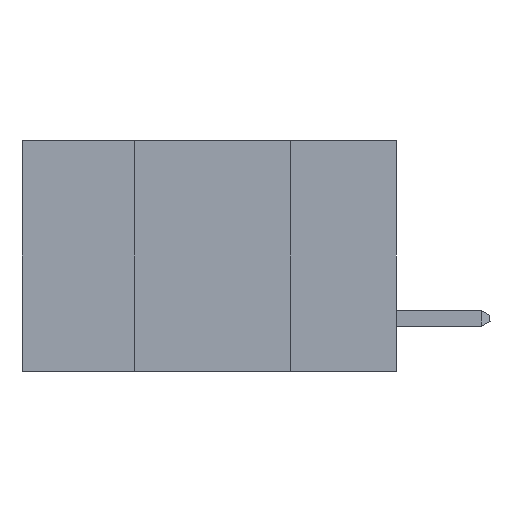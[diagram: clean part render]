
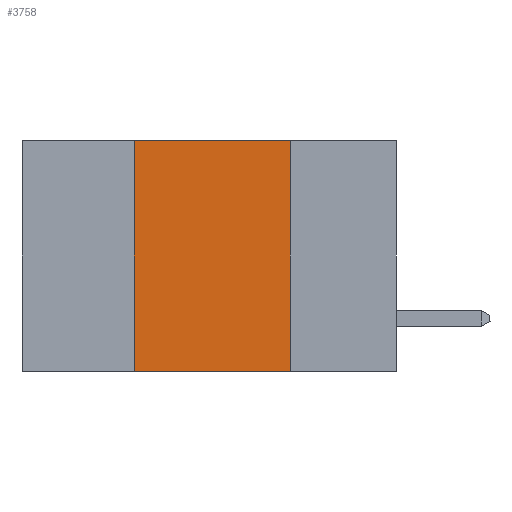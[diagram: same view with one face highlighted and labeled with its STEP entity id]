
A CAD part, left-side view. The second image highlights one B-rep face of the part: STEP entity #3758.
In plain terms, the highlighted planar face has unit normal (-1, 0, 0).
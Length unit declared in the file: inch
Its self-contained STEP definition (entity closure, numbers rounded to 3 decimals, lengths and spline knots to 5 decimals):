
#386 = LINE ( 'NONE', #14880, #13480 ) ;
#495 = DIRECTION ( 'NONE',  ( 0., 0., 1. ) ) ;
#1566 = VECTOR ( 'NONE', #15967, 39.37008 ) ;
#2163 = DIRECTION ( 'NONE',  ( 0., -1., 0. ) ) ;
#2364 = VECTOR ( 'NONE', #2163, 39.37008 ) ;
#2517 = EDGE_LOOP ( 'NONE', ( #6542, #15307, #7338, #2633 ) ) ;
#2633 = ORIENTED_EDGE ( 'NONE', *, *, #7974, .T. ) ;
#3292 = DIRECTION ( 'NONE',  ( 1., 0., 0. ) ) ;
#3332 = VERTEX_POINT ( 'NONE', #13618 ) ;
#3379 = DIRECTION ( 'NONE',  ( 0., 0., -1. ) ) ;
#3758 = ADVANCED_FACE ( 'NONE', ( #7719 ), #9245, .F. ) ;
#4169 = VERTEX_POINT ( 'NONE', #14864 ) ;
#4485 = CARTESIAN_POINT ( 'NONE',  ( 0., 0.6, 0. ) ) ;
#4573 = CARTESIAN_POINT ( 'NONE',  ( 0., 0.17, 0. ) ) ;
#5188 = EDGE_CURVE ( 'NONE', #4169, #11211, #386, .T. ) ;
#5223 = CARTESIAN_POINT ( 'NONE',  ( 0., 0.42, 0. ) ) ;
#6510 = CARTESIAN_POINT ( 'NONE',  ( 0., 0.6, 0. ) ) ;
#6542 = ORIENTED_EDGE ( 'NONE', *, *, #9385, .F. ) ;
#7338 = ORIENTED_EDGE ( 'NONE', *, *, #5188, .F. ) ;
#7719 = FACE_OUTER_BOUND ( 'NONE', #2517, .T. ) ;
#7974 = EDGE_CURVE ( 'NONE', #4169, #3332, #15461, .T. ) ;
#8826 = AXIS2_PLACEMENT_3D ( 'NONE', #4485, #3292, #3379 ) ;
#9245 = PLANE ( 'NONE',  #8826 ) ;
#9385 = EDGE_CURVE ( 'NONE', #10269, #3332, #10312, .T. ) ;
#9927 = VECTOR ( 'NONE', #11454, 39.37008 ) ;
#10269 = VERTEX_POINT ( 'NONE', #4573 ) ;
#10312 = LINE ( 'NONE', #15921, #9927 ) ;
#11121 = CARTESIAN_POINT ( 'NONE',  ( 0., 0.6, -0.37 ) ) ;
#11211 = VERTEX_POINT ( 'NONE', #5223 ) ;
#11454 = DIRECTION ( 'NONE',  ( 0., 0., -1. ) ) ;
#11773 = LINE ( 'NONE', #6510, #1566 ) ;
#13480 = VECTOR ( 'NONE', #495, 39.37008 ) ;
#13618 = CARTESIAN_POINT ( 'NONE',  ( 0., 0.17, -0.37 ) ) ;
#14278 = EDGE_CURVE ( 'NONE', #11211, #10269, #11773, .T. ) ;
#14864 = CARTESIAN_POINT ( 'NONE',  ( 0., 0.42, -0.37 ) ) ;
#14880 = CARTESIAN_POINT ( 'NONE',  ( 0., 0.42, 0. ) ) ;
#15307 = ORIENTED_EDGE ( 'NONE', *, *, #14278, .F. ) ;
#15461 = LINE ( 'NONE', #11121, #2364 ) ;
#15921 = CARTESIAN_POINT ( 'NONE',  ( 0., 0.17, 0. ) ) ;
#15967 = DIRECTION ( 'NONE',  ( 0., -1., 0. ) ) ;
